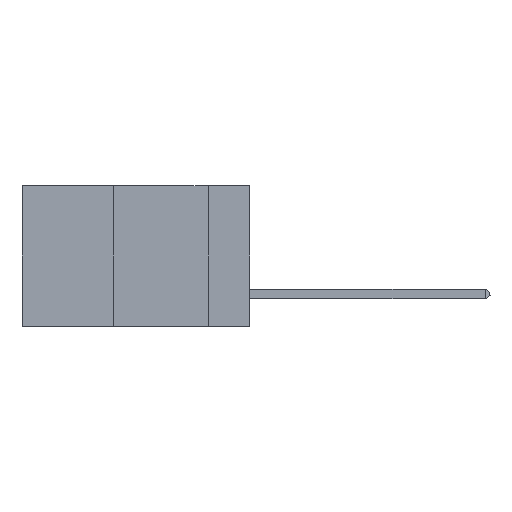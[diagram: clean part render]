
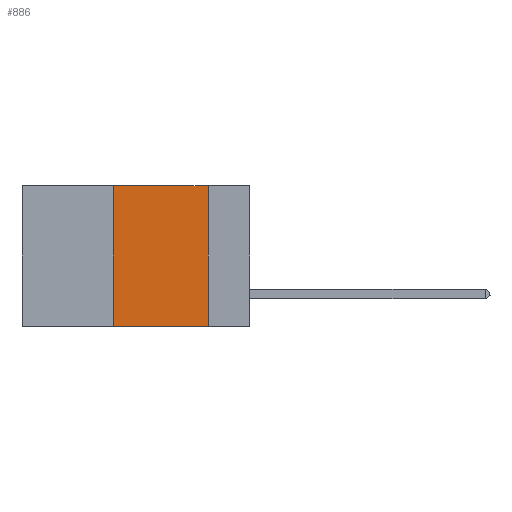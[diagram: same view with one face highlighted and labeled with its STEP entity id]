
A CAD part, left-side view. The second image highlights one B-rep face of the part: STEP entity #886.
In plain terms, the highlighted planar face has unit normal (-1, 0, 0).
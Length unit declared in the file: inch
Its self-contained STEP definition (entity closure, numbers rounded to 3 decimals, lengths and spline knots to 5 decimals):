
#886 = ADVANCED_FACE ( 'NONE', ( #27396 ), #10767, .F. ) ;
#1795 = DIRECTION ( 'NONE',  ( 0., 0., -1. ) ) ;
#2189 = CARTESIAN_POINT ( 'NONE',  ( 0., 0.11, 0. ) ) ;
#2237 = CARTESIAN_POINT ( 'NONE',  ( 0., 0.36, -0.37 ) ) ;
#2409 = VECTOR ( 'NONE', #28470, 39.37008 ) ;
#3876 = AXIS2_PLACEMENT_3D ( 'NONE', #35463, #14132, #1795 ) ;
#5651 = CARTESIAN_POINT ( 'NONE',  ( 0., 0.36, 0. ) ) ;
#5881 = LINE ( 'NONE', #35499, #15469 ) ;
#6418 = ORIENTED_EDGE ( 'NONE', *, *, #28697, .T. ) ;
#9711 = VECTOR ( 'NONE', #24296, 39.37008 ) ;
#10157 = ORIENTED_EDGE ( 'NONE', *, *, #39247, .F. ) ;
#10673 = CARTESIAN_POINT ( 'NONE',  ( 0., 0.6, 0. ) ) ;
#10767 = PLANE ( 'NONE',  #3876 ) ;
#10830 = LINE ( 'NONE', #28606, #2409 ) ;
#13811 = VERTEX_POINT ( 'NONE', #2237 ) ;
#14132 = DIRECTION ( 'NONE',  ( 1., 0., 0. ) ) ;
#15469 = VECTOR ( 'NONE', #20371, 39.37008 ) ;
#16320 = LINE ( 'NONE', #10673, #24074 ) ;
#18064 = VERTEX_POINT ( 'NONE', #25607 ) ;
#20371 = DIRECTION ( 'NONE',  ( 0., -1., 0. ) ) ;
#21668 = ORIENTED_EDGE ( 'NONE', *, *, #37213, .F. ) ;
#22239 = LINE ( 'NONE', #36852, #9711 ) ;
#24074 = VECTOR ( 'NONE', #26161, 39.37008 ) ;
#24296 = DIRECTION ( 'NONE',  ( 0., 0., 1. ) ) ;
#25607 = CARTESIAN_POINT ( 'NONE',  ( 0., 0.11, -0.37 ) ) ;
#26161 = DIRECTION ( 'NONE',  ( 0., -1., 0. ) ) ;
#27396 = FACE_OUTER_BOUND ( 'NONE', #34786, .T. ) ;
#28470 = DIRECTION ( 'NONE',  ( 0., 0., -1. ) ) ;
#28606 = CARTESIAN_POINT ( 'NONE',  ( 0., 0.11, 0. ) ) ;
#28697 = EDGE_CURVE ( 'NONE', #13811, #18064, #5881, .T. ) ;
#29569 = ORIENTED_EDGE ( 'NONE', *, *, #32299, .F. ) ;
#29641 = VERTEX_POINT ( 'NONE', #5651 ) ;
#32299 = EDGE_CURVE ( 'NONE', #35280, #18064, #10830, .T. ) ;
#34786 = EDGE_LOOP ( 'NONE', ( #29569, #10157, #21668, #6418 ) ) ;
#35280 = VERTEX_POINT ( 'NONE', #2189 ) ;
#35463 = CARTESIAN_POINT ( 'NONE',  ( 0., 0.6, 0. ) ) ;
#35499 = CARTESIAN_POINT ( 'NONE',  ( 0., 0.6, -0.37 ) ) ;
#36852 = CARTESIAN_POINT ( 'NONE',  ( 0., 0.36, 0. ) ) ;
#37213 = EDGE_CURVE ( 'NONE', #13811, #29641, #22239, .T. ) ;
#39247 = EDGE_CURVE ( 'NONE', #29641, #35280, #16320, .T. ) ;
